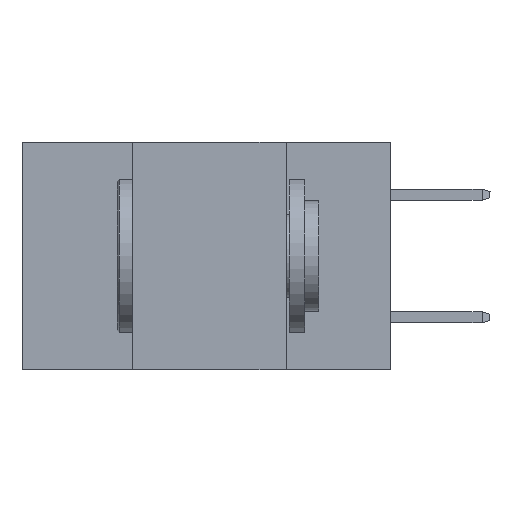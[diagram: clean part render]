
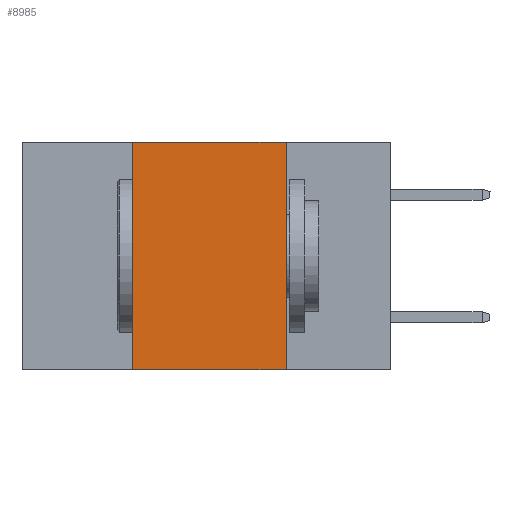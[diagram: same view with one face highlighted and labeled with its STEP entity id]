
A CAD part, left-side view. The second image highlights one B-rep face of the part: STEP entity #8985.
In plain terms, the highlighted planar face has unit normal (-1, 0, 0).
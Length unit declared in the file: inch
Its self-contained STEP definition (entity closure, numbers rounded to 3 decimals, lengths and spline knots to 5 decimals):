
#57 = CARTESIAN_POINT ( 'NONE',  ( 0., 0.42, -0.37 ) ) ;
#330 = CARTESIAN_POINT ( 'NONE',  ( 0., 0.6, 0. ) ) ;
#405 = DIRECTION ( 'NONE',  ( 0., -1., 0. ) ) ;
#1208 = ORIENTED_EDGE ( 'NONE', *, *, #3764, .F. ) ;
#1245 = FACE_OUTER_BOUND ( 'NONE', #17586, .T. ) ;
#1558 = CARTESIAN_POINT ( 'NONE',  ( 0., 0.6, 0. ) ) ;
#2529 = CARTESIAN_POINT ( 'NONE',  ( 0., 0.17, -0.37 ) ) ;
#3159 = LINE ( 'NONE', #5377, #17567 ) ;
#3764 = EDGE_CURVE ( 'NONE', #20545, #5361, #12437, .T. ) ;
#4744 = LINE ( 'NONE', #12673, #11143 ) ;
#5023 = DIRECTION ( 'NONE',  ( 1., 0., 0. ) ) ;
#5025 = EDGE_CURVE ( 'NONE', #20292, #20545, #10829, .T. ) ;
#5304 = ORIENTED_EDGE ( 'NONE', *, *, #19121, .F. ) ;
#5361 = VERTEX_POINT ( 'NONE', #13509 ) ;
#5377 = CARTESIAN_POINT ( 'NONE',  ( 0., 0.17, 0. ) ) ;
#5616 = CARTESIAN_POINT ( 'NONE',  ( 0., 0.42, 0. ) ) ;
#6305 = VECTOR ( 'NONE', #405, 39.37008 ) ;
#7800 = CARTESIAN_POINT ( 'NONE',  ( 0., 0.42, 0. ) ) ;
#8254 = ORIENTED_EDGE ( 'NONE', *, *, #5025, .F. ) ;
#8985 = ADVANCED_FACE ( 'NONE', ( #1245 ), #11572, .F. ) ;
#9208 = EDGE_CURVE ( 'NONE', #20292, #10503, #4744, .T. ) ;
#9518 = VECTOR ( 'NONE', #14498, 39.37008 ) ;
#10503 = VERTEX_POINT ( 'NONE', #2529 ) ;
#10829 = LINE ( 'NONE', #7800, #9518 ) ;
#11143 = VECTOR ( 'NONE', #14186, 39.37008 ) ;
#11572 = PLANE ( 'NONE',  #19059 ) ;
#12437 = LINE ( 'NONE', #330, #6305 ) ;
#12673 = CARTESIAN_POINT ( 'NONE',  ( 0., 0.6, -0.37 ) ) ;
#13385 = ORIENTED_EDGE ( 'NONE', *, *, #9208, .T. ) ;
#13509 = CARTESIAN_POINT ( 'NONE',  ( 0., 0.17, 0. ) ) ;
#14186 = DIRECTION ( 'NONE',  ( 0., -1., 0. ) ) ;
#14498 = DIRECTION ( 'NONE',  ( 0., 0., 1. ) ) ;
#14763 = DIRECTION ( 'NONE',  ( 0., 0., -1. ) ) ;
#15291 = DIRECTION ( 'NONE',  ( 0., 0., -1. ) ) ;
#17567 = VECTOR ( 'NONE', #14763, 39.37008 ) ;
#17586 = EDGE_LOOP ( 'NONE', ( #5304, #1208, #8254, #13385 ) ) ;
#19059 = AXIS2_PLACEMENT_3D ( 'NONE', #1558, #5023, #15291 ) ;
#19121 = EDGE_CURVE ( 'NONE', #5361, #10503, #3159, .T. ) ;
#20292 = VERTEX_POINT ( 'NONE', #57 ) ;
#20545 = VERTEX_POINT ( 'NONE', #5616 ) ;
